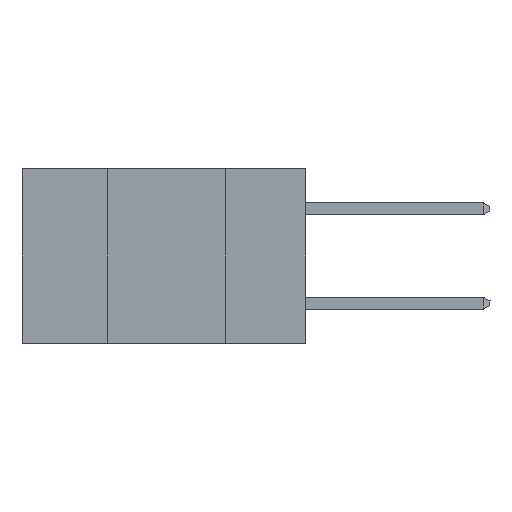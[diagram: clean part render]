
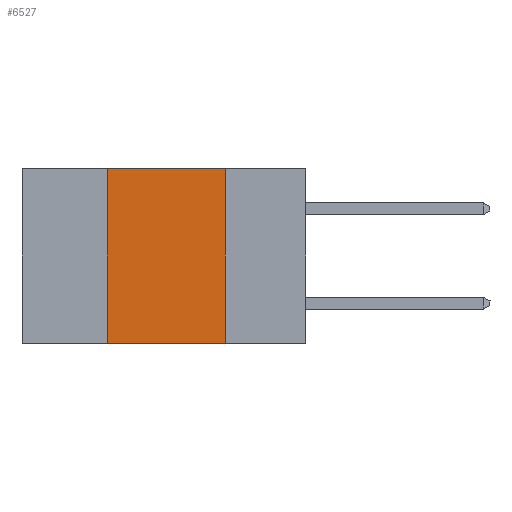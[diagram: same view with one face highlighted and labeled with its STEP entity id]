
A CAD part, left-side view. The second image highlights one B-rep face of the part: STEP entity #6527.
In plain terms, the highlighted planar face has unit normal (-1, 0, 0).
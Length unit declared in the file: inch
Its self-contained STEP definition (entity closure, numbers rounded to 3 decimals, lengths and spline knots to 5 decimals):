
#1894 = ORIENTED_EDGE ( 'NONE', *, *, #11773, .F. ) ;
#2218 = DIRECTION ( 'NONE',  ( 1., 0., 0. ) ) ;
#2271 = PLANE ( 'NONE',  #9535 ) ;
#2898 = ORIENTED_EDGE ( 'NONE', *, *, #4534, .F. ) ;
#2967 = LINE ( 'NONE', #14931, #5577 ) ;
#3875 = EDGE_LOOP ( 'NONE', ( #2898, #1894, #15987, #10285 ) ) ;
#4117 = CARTESIAN_POINT ( 'NONE',  ( 0., 0.17, -0.37 ) ) ;
#4132 = CARTESIAN_POINT ( 'NONE',  ( 0., 0.6, -0.37 ) ) ;
#4512 = CARTESIAN_POINT ( 'NONE',  ( 0., 0.6, 0. ) ) ;
#4534 = EDGE_CURVE ( 'NONE', #9752, #15207, #2967, .T. ) ;
#4661 = DIRECTION ( 'NONE',  ( 0., 0., -1. ) ) ;
#4814 = LINE ( 'NONE', #4132, #11144 ) ;
#5471 = VERTEX_POINT ( 'NONE', #9162 ) ;
#5577 = VECTOR ( 'NONE', #9874, 39.37008 ) ;
#5942 = LINE ( 'NONE', #4512, #13449 ) ;
#6494 = EDGE_CURVE ( 'NONE', #12045, #5471, #7492, .T. ) ;
#6527 = ADVANCED_FACE ( 'NONE', ( #10235 ), #2271, .F. ) ;
#7492 = LINE ( 'NONE', #15988, #13014 ) ;
#8149 = CARTESIAN_POINT ( 'NONE',  ( 0., 0.17, 0. ) ) ;
#9154 = DIRECTION ( 'NONE',  ( 0., -1., 0. ) ) ;
#9162 = CARTESIAN_POINT ( 'NONE',  ( 0., 0.42, 0. ) ) ;
#9535 = AXIS2_PLACEMENT_3D ( 'NONE', #14742, #2218, #4661 ) ;
#9752 = VERTEX_POINT ( 'NONE', #8149 ) ;
#9874 = DIRECTION ( 'NONE',  ( 0., 0., -1. ) ) ;
#10235 = FACE_OUTER_BOUND ( 'NONE', #3875, .T. ) ;
#10285 = ORIENTED_EDGE ( 'NONE', *, *, #16383, .T. ) ;
#11144 = VECTOR ( 'NONE', #9154, 39.37008 ) ;
#11773 = EDGE_CURVE ( 'NONE', #5471, #9752, #5942, .T. ) ;
#12045 = VERTEX_POINT ( 'NONE', #14081 ) ;
#12257 = DIRECTION ( 'NONE',  ( 0., -1., 0. ) ) ;
#13014 = VECTOR ( 'NONE', #16156, 39.37008 ) ;
#13449 = VECTOR ( 'NONE', #12257, 39.37008 ) ;
#14081 = CARTESIAN_POINT ( 'NONE',  ( 0., 0.42, -0.37 ) ) ;
#14742 = CARTESIAN_POINT ( 'NONE',  ( 0., 0.6, 0. ) ) ;
#14931 = CARTESIAN_POINT ( 'NONE',  ( 0., 0.17, 0. ) ) ;
#15207 = VERTEX_POINT ( 'NONE', #4117 ) ;
#15987 = ORIENTED_EDGE ( 'NONE', *, *, #6494, .F. ) ;
#15988 = CARTESIAN_POINT ( 'NONE',  ( 0., 0.42, 0. ) ) ;
#16156 = DIRECTION ( 'NONE',  ( 0., 0., 1. ) ) ;
#16383 = EDGE_CURVE ( 'NONE', #12045, #15207, #4814, .T. ) ;
